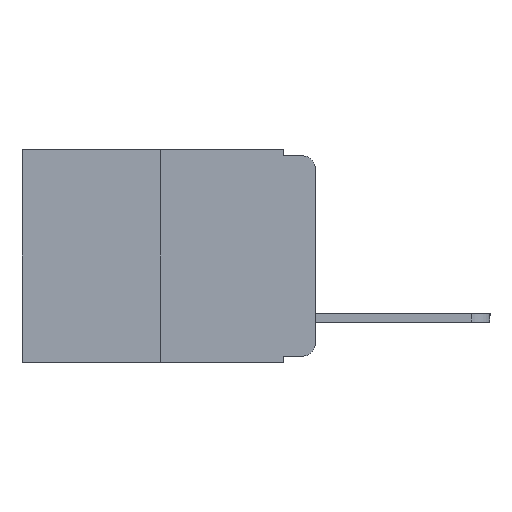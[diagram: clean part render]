
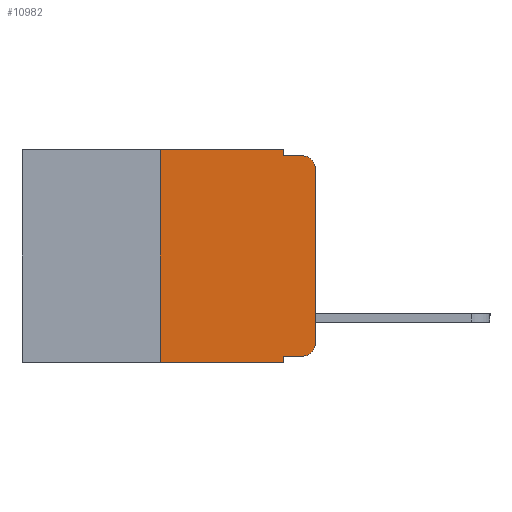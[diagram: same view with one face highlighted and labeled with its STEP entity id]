
A CAD part, left-side view. The second image highlights one B-rep face of the part: STEP entity #10982.
In plain terms, the highlighted planar face has unit normal (-1, 0, 0).
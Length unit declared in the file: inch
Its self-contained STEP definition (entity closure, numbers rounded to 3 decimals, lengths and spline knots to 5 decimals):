
#1 = DIRECTION ( 'NONE',  ( 0., 0., -1. ) ) ;
#123 = VECTOR ( 'NONE', #4231, 39.37008 ) ;
#172 = DIRECTION ( 'NONE',  ( 0., 0., 1. ) ) ;
#1457 = VERTEX_POINT ( 'NONE', #4146 ) ;
#1502 = VERTEX_POINT ( 'NONE', #2835 ) ;
#1520 = VECTOR ( 'NONE', #2756, 39.37008 ) ;
#1696 = CARTESIAN_POINT ( 'NONE',  ( 0., 0.051, 0. ) ) ;
#1710 = DIRECTION ( 'NONE',  ( 1., 0., 0. ) ) ;
#1945 = ORIENTED_EDGE ( 'NONE', *, *, #7642, .F. ) ;
#2361 = VERTEX_POINT ( 'NONE', #10697 ) ;
#2399 = CARTESIAN_POINT ( 'NONE',  ( 0., 0.02, -0.03 ) ) ;
#2437 = VERTEX_POINT ( 'NONE', #10373 ) ;
#2646 = DIRECTION ( 'NONE',  ( 0., 0., -1. ) ) ;
#2664 = LINE ( 'NONE', #7300, #7298 ) ;
#2684 = LINE ( 'NONE', #9605, #123 ) ;
#2756 = DIRECTION ( 'NONE',  ( 0., 0., 1. ) ) ;
#2823 = ORIENTED_EDGE ( 'NONE', *, *, #5867, .T. ) ;
#2835 = CARTESIAN_POINT ( 'NONE',  ( 0., 0.051, -0.01 ) ) ;
#3327 = LINE ( 'NONE', #10240, #8491 ) ;
#3352 = DIRECTION ( 'NONE',  ( 0., 0., -1. ) ) ;
#3741 = DIRECTION ( 'NONE',  ( -1., 0., 0. ) ) ;
#4146 = CARTESIAN_POINT ( 'NONE',  ( 0., 0., -0.313 ) ) ;
#4200 = AXIS2_PLACEMENT_3D ( 'NONE', #5480, #1710, #8179 ) ;
#4231 = DIRECTION ( 'NONE',  ( 0., -1., 0. ) ) ;
#4267 = DIRECTION ( 'NONE',  ( 0., -1., 0. ) ) ;
#4346 = CARTESIAN_POINT ( 'NONE',  ( 0., 0.473, 0. ) ) ;
#4396 = CARTESIAN_POINT ( 'NONE',  ( 0., 0.25, 0. ) ) ;
#4788 = CARTESIAN_POINT ( 'NONE',  ( 0., 0.051, 0. ) ) ;
#4838 = VERTEX_POINT ( 'NONE', #4396 ) ;
#4876 = VECTOR ( 'NONE', #4267, 39.37008 ) ;
#5097 = EDGE_CURVE ( 'NONE', #9861, #1502, #11482, .T. ) ;
#5259 = EDGE_CURVE ( 'NONE', #9469, #4838, #3327, .T. ) ;
#5343 = EDGE_CURVE ( 'NONE', #2361, #9660, #7356, .T. ) ;
#5480 = CARTESIAN_POINT ( 'NONE',  ( 0., 0.473, 0. ) ) ;
#5867 = EDGE_CURVE ( 'NONE', #9660, #1457, #6761, .T. ) ;
#6039 = ORIENTED_EDGE ( 'NONE', *, *, #6552, .T. ) ;
#6185 = CARTESIAN_POINT ( 'NONE',  ( 0., 0.051, -0.343 ) ) ;
#6202 = EDGE_LOOP ( 'NONE', ( #6039, #10629, #6601, #8956, #1945, #11432, #9492, #7442, #9764, #2823 ) ) ;
#6550 = AXIS2_PLACEMENT_3D ( 'NONE', #9134, #3741, #9987 ) ;
#6552 = EDGE_CURVE ( 'NONE', #1457, #7603, #9103, .T. ) ;
#6588 = VECTOR ( 'NONE', #8891, 39.37008 ) ;
#6601 = ORIENTED_EDGE ( 'NONE', *, *, #9157, .F. ) ;
#6761 = CIRCLE ( 'NONE', #6550, 0.02 ) ;
#6880 = DIRECTION ( 'NONE',  ( 0., -1., 0. ) ) ;
#6886 = LINE ( 'NONE', #4346, #6588 ) ;
#6894 = EDGE_CURVE ( 'NONE', #9469, #8338, #2684, .T. ) ;
#7278 = PLANE ( 'NONE',  #4200 ) ;
#7298 = VECTOR ( 'NONE', #2646, 39.37008 ) ;
#7300 = CARTESIAN_POINT ( 'NONE',  ( 0., 0.051, 0. ) ) ;
#7356 = LINE ( 'NONE', #7776, #9395 ) ;
#7387 = CIRCLE ( 'NONE', #10297, 0.02 ) ;
#7442 = ORIENTED_EDGE ( 'NONE', *, *, #7802, .F. ) ;
#7497 = CARTESIAN_POINT ( 'NONE',  ( 0., 0.25, -0.343 ) ) ;
#7542 = LINE ( 'NONE', #8792, #4876 ) ;
#7603 = VERTEX_POINT ( 'NONE', #9670 ) ;
#7642 = EDGE_CURVE ( 'NONE', #4838, #9861, #6886, .T. ) ;
#7729 = CARTESIAN_POINT ( 'NONE',  ( 0., 0.02, -0.333 ) ) ;
#7776 = CARTESIAN_POINT ( 'NONE',  ( 0., 0.051, -0.333 ) ) ;
#7802 = EDGE_CURVE ( 'NONE', #2361, #8338, #2664, .T. ) ;
#8179 = DIRECTION ( 'NONE',  ( 0., 0., -1. ) ) ;
#8338 = VERTEX_POINT ( 'NONE', #6185 ) ;
#8491 = VECTOR ( 'NONE', #172, 39.37008 ) ;
#8792 = CARTESIAN_POINT ( 'NONE',  ( 0., 0.051, -0.01 ) ) ;
#8811 = DIRECTION ( 'NONE',  ( -1., 0., 0. ) ) ;
#8891 = DIRECTION ( 'NONE',  ( 0., -1., 0. ) ) ;
#8956 = ORIENTED_EDGE ( 'NONE', *, *, #5097, .F. ) ;
#9103 = LINE ( 'NONE', #11598, #1520 ) ;
#9134 = CARTESIAN_POINT ( 'NONE',  ( 0., 0.02, -0.313 ) ) ;
#9157 = EDGE_CURVE ( 'NONE', #1502, #2437, #7542, .T. ) ;
#9395 = VECTOR ( 'NONE', #6880, 39.37008 ) ;
#9469 = VERTEX_POINT ( 'NONE', #7497 ) ;
#9492 = ORIENTED_EDGE ( 'NONE', *, *, #6894, .T. ) ;
#9539 = VECTOR ( 'NONE', #1, 39.37008 ) ;
#9605 = CARTESIAN_POINT ( 'NONE',  ( 0., 0.473, -0.343 ) ) ;
#9660 = VERTEX_POINT ( 'NONE', #7729 ) ;
#9670 = CARTESIAN_POINT ( 'NONE',  ( 0., 0., -0.03 ) ) ;
#9764 = ORIENTED_EDGE ( 'NONE', *, *, #5343, .T. ) ;
#9805 = EDGE_CURVE ( 'NONE', #7603, #2437, #7387, .T. ) ;
#9861 = VERTEX_POINT ( 'NONE', #1696 ) ;
#9987 = DIRECTION ( 'NONE',  ( 0., 0., -1. ) ) ;
#10240 = CARTESIAN_POINT ( 'NONE',  ( 0., 0.25, 0. ) ) ;
#10297 = AXIS2_PLACEMENT_3D ( 'NONE', #2399, #8811, #3352 ) ;
#10373 = CARTESIAN_POINT ( 'NONE',  ( 0., 0.02, -0.01 ) ) ;
#10443 = FACE_OUTER_BOUND ( 'NONE', #6202, .T. ) ;
#10629 = ORIENTED_EDGE ( 'NONE', *, *, #9805, .T. ) ;
#10697 = CARTESIAN_POINT ( 'NONE',  ( 0., 0.051, -0.333 ) ) ;
#10982 = ADVANCED_FACE ( 'NONE', ( #10443 ), #7278, .F. ) ;
#11432 = ORIENTED_EDGE ( 'NONE', *, *, #5259, .F. ) ;
#11482 = LINE ( 'NONE', #4788, #9539 ) ;
#11598 = CARTESIAN_POINT ( 'NONE',  ( 0., 0., 0. ) ) ;
